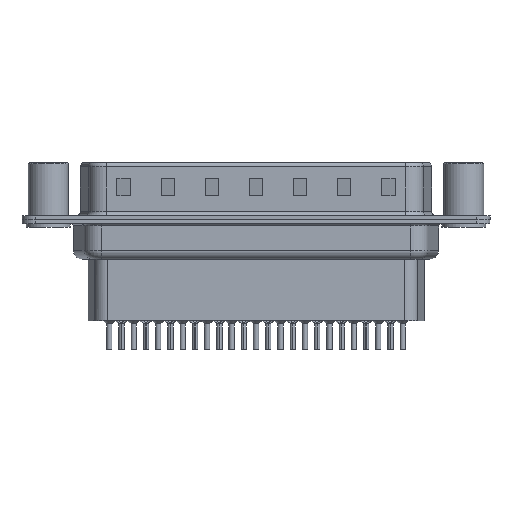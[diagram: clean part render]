
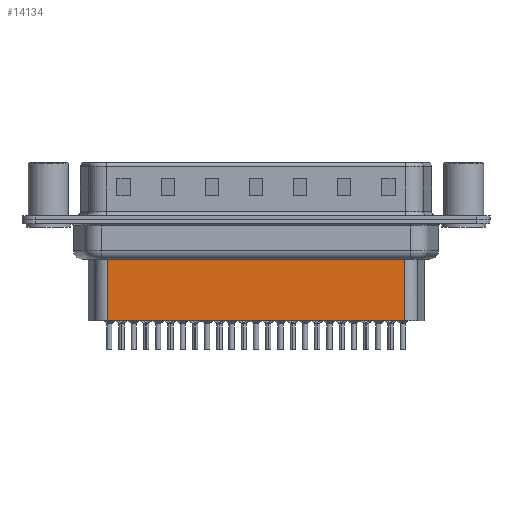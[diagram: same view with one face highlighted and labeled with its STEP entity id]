
A CAD part, front view. The second image highlights one B-rep face of the part: STEP entity #14134.
In plain terms, the highlighted planar face has unit normal (0, -1, 0).
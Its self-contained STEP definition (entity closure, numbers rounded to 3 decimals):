
#99 = DIRECTION ( 'NONE',  ( 0., -1., 0. ) ) ;
#118 = EDGE_LOOP ( 'NONE', ( #12674, #3602, #19009, #15306 ) ) ;
#427 = DIRECTION ( 'NONE',  ( -1., 0., 0. ) ) ;
#435 = DIRECTION ( 'NONE',  ( 0., 0., -1. ) ) ;
#438 = CARTESIAN_POINT ( 'NONE',  ( 6.706, -3.5, -3.1 ) ) ;
#1101 = LINE ( 'NONE', #18774, #21159 ) ;
#1666 = EDGE_CURVE ( 'NONE', #21016, #2399, #2627, .T. ) ;
#2396 = CARTESIAN_POINT ( 'NONE',  ( 6.706, -3.5, -11.45 ) ) ;
#2399 = VERTEX_POINT ( 'NONE', #16992 ) ;
#2501 = LINE ( 'NONE', #25643, #12634 ) ;
#2627 = LINE ( 'NONE', #438, #7413 ) ;
#3073 = LINE ( 'NONE', #2396, #14440 ) ;
#3602 = ORIENTED_EDGE ( 'NONE', *, *, #5299, .T. ) ;
#5299 = EDGE_CURVE ( 'NONE', #15106, #21016, #2501, .T. ) ;
#6567 = AXIS2_PLACEMENT_3D ( 'NONE', #10147, #99, #14225 ) ;
#7413 = VECTOR ( 'NONE', #435, 1000. ) ;
#9198 = VERTEX_POINT ( 'NONE', #20913 ) ;
#9220 = CARTESIAN_POINT ( 'NONE',  ( 40.344, -3.5, -4.097 ) ) ;
#10147 = CARTESIAN_POINT ( 'NONE',  ( 6.706, -3.5, -3.1 ) ) ;
#10346 = EDGE_CURVE ( 'NONE', #9198, #2399, #3073, .T. ) ;
#12170 = PLANE ( 'NONE',  #6567 ) ;
#12634 = VECTOR ( 'NONE', #24196, 1000. ) ;
#12674 = ORIENTED_EDGE ( 'NONE', *, *, #14335, .F. ) ;
#14134 = ADVANCED_FACE ( 'NONE', ( #20869 ), #12170, .T. ) ;
#14225 = DIRECTION ( 'NONE',  ( 1., 0., 0. ) ) ;
#14335 = EDGE_CURVE ( 'NONE', #15106, #9198, #1101, .T. ) ;
#14440 = VECTOR ( 'NONE', #427, 1000. ) ;
#15106 = VERTEX_POINT ( 'NONE', #9220 ) ;
#15306 = ORIENTED_EDGE ( 'NONE', *, *, #10346, .F. ) ;
#16758 = DIRECTION ( 'NONE',  ( 0., 0., -1. ) ) ;
#16992 = CARTESIAN_POINT ( 'NONE',  ( 6.706, -3.5, -11.45 ) ) ;
#18774 = CARTESIAN_POINT ( 'NONE',  ( 40.344, -3.5, -3.1 ) ) ;
#19009 = ORIENTED_EDGE ( 'NONE', *, *, #1666, .T. ) ;
#20869 = FACE_OUTER_BOUND ( 'NONE', #118, .T. ) ;
#20913 = CARTESIAN_POINT ( 'NONE',  ( 40.344, -3.5, -11.45 ) ) ;
#21016 = VERTEX_POINT ( 'NONE', #24243 ) ;
#21159 = VECTOR ( 'NONE', #16758, 1000. ) ;
#24196 = DIRECTION ( 'NONE',  ( -1., 0., 0. ) ) ;
#24243 = CARTESIAN_POINT ( 'NONE',  ( 6.706, -3.5, -4.097 ) ) ;
#25643 = CARTESIAN_POINT ( 'NONE',  ( 6.459, -3.5, -4.097 ) ) ;
